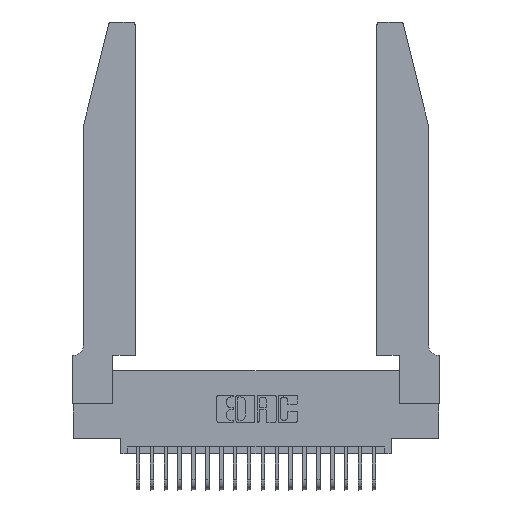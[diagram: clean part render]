
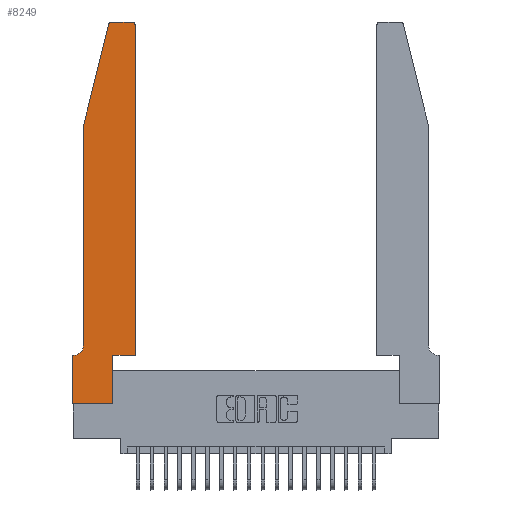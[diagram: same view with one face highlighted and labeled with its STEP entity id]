
A CAD part, top view. The second image highlights one B-rep face of the part: STEP entity #8249.
In plain terms, the highlighted planar face has unit normal (0, 0, 1).
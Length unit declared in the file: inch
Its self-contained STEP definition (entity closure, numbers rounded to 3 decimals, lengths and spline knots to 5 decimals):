
#25 = VERTEX_POINT ( 'NONE', #424 ) ;
#424 = CARTESIAN_POINT ( 'NONE',  ( 0.0055, 0.35, 0.37 ) ) ;
#788 = VERTEX_POINT ( 'NONE', #925 ) ;
#873 = EDGE_CURVE ( 'NONE', #8035, #13898, #9835, .T. ) ;
#921 = CARTESIAN_POINT ( 'NONE',  ( 0.2865, 0.35, 0.37 ) ) ;
#925 = CARTESIAN_POINT ( 'NONE',  ( 0.0755, 2., 0.37 ) ) ;
#930 = LINE ( 'NONE', #13418, #6035 ) ;
#1187 = ORIENTED_EDGE ( 'NONE', *, *, #9232, .T. ) ;
#1329 = DIRECTION ( 'NONE',  ( 0., 0., 1. ) ) ;
#1431 = EDGE_CURVE ( 'NONE', #19298, #11202, #3705, .T. ) ;
#1571 = CIRCLE ( 'NONE', #3192, 0.07 ) ;
#1923 = ORIENTED_EDGE ( 'NONE', *, *, #21018, .T. ) ;
#2057 = CARTESIAN_POINT ( 'NONE',  ( 0.4205, 2.75, 0.37 ) ) ;
#2669 = DIRECTION ( 'NONE',  ( 0., 1., 0. ) ) ;
#2806 = CARTESIAN_POINT ( 'NONE',  ( 0., 0.35, 0.37 ) ) ;
#3167 = VECTOR ( 'NONE', #20704, 39.37008 ) ;
#3180 = VERTEX_POINT ( 'NONE', #6716 ) ;
#3192 = AXIS2_PLACEMENT_3D ( 'NONE', #5181, #16887, #6897 ) ;
#3321 = DIRECTION ( 'NONE',  ( -1., 0., 0. ) ) ;
#3704 = CARTESIAN_POINT ( 'NONE',  ( 0.0755, 0.42, 0.37 ) ) ;
#3705 = LINE ( 'NONE', #14028, #3167 ) ;
#3751 = ORIENTED_EDGE ( 'NONE', *, *, #15415, .T. ) ;
#3829 = CARTESIAN_POINT ( 'NONE',  ( 0.4505, 0.35, 0.37 ) ) ;
#4126 = ORIENTED_EDGE ( 'NONE', *, *, #1431, .T. ) ;
#4267 = LINE ( 'NONE', #21011, #12687 ) ;
#4289 = DIRECTION ( 'NONE',  ( 0., 1., 0. ) ) ;
#4450 = AXIS2_PLACEMENT_3D ( 'NONE', #18983, #11532, #5230 ) ;
#4465 = CARTESIAN_POINT ( 'NONE',  ( 0., 0., 0.37 ) ) ;
#4555 = DIRECTION ( 'NONE',  ( 1., 0., 0. ) ) ;
#4570 = DIRECTION ( 'NONE',  ( 0., -1., 0. ) ) ;
#5181 = CARTESIAN_POINT ( 'NONE',  ( 0.0055, 0.42, 0.37 ) ) ;
#5230 = DIRECTION ( 'NONE',  ( 1., 0., 0. ) ) ;
#5267 = CARTESIAN_POINT ( 'NONE',  ( 0.0755, 0.35, 0.37 ) ) ;
#5274 = CARTESIAN_POINT ( 'NONE',  ( 0.284, 2.75, 0.37 ) ) ;
#6035 = VECTOR ( 'NONE', #3321, 39.37008 ) ;
#6087 = VERTEX_POINT ( 'NONE', #16178 ) ;
#6157 = DIRECTION ( 'NONE',  ( 0., -1., 0. ) ) ;
#6173 = PLANE ( 'NONE',  #8786 ) ;
#6716 = CARTESIAN_POINT ( 'NONE',  ( 0.2865, 0.35, 0.37 ) ) ;
#6897 = DIRECTION ( 'NONE',  ( -1., 0., 0. ) ) ;
#6988 = DIRECTION ( 'NONE',  ( -1., 0., 0. ) ) ;
#7423 = LINE ( 'NONE', #5267, #15754 ) ;
#7654 = VECTOR ( 'NONE', #6157, 39.37008 ) ;
#8035 = VERTEX_POINT ( 'NONE', #20699 ) ;
#8249 = ADVANCED_FACE ( 'NONE', ( #14577 ), #6173, .T. ) ;
#8595 = ORIENTED_EDGE ( 'NONE', *, *, #15744, .T. ) ;
#8786 = AXIS2_PLACEMENT_3D ( 'NONE', #2806, #14583, #4555 ) ;
#8890 = ORIENTED_EDGE ( 'NONE', *, *, #12503, .T. ) ;
#8979 = EDGE_CURVE ( 'NONE', #18994, #13188, #19507, .T. ) ;
#9232 = EDGE_CURVE ( 'NONE', #3180, #6087, #14841, .T. ) ;
#9474 = EDGE_CURVE ( 'NONE', #788, #10810, #11680, .T. ) ;
#9787 = VECTOR ( 'NONE', #2669, 39.37008 ) ;
#9819 = ORIENTED_EDGE ( 'NONE', *, *, #873, .T. ) ;
#9835 = CIRCLE ( 'NONE', #4450, 0.03 ) ;
#9926 = CARTESIAN_POINT ( 'NONE',  ( 0.0755, 2., 0.37 ) ) ;
#10230 = CARTESIAN_POINT ( 'NONE',  ( 0., 0.35, 0.37 ) ) ;
#10776 = LINE ( 'NONE', #9926, #18576 ) ;
#10810 = VERTEX_POINT ( 'NONE', #3704 ) ;
#11202 = VERTEX_POINT ( 'NONE', #19853 ) ;
#11277 = AXIS2_PLACEMENT_3D ( 'NONE', #11471, #1329, #13193 ) ;
#11471 = CARTESIAN_POINT ( 'NONE',  ( 0.284, 2.72, 0.37 ) ) ;
#11532 = DIRECTION ( 'NONE',  ( 0., 0., 1. ) ) ;
#11680 = LINE ( 'NONE', #21210, #19488 ) ;
#12456 = ORIENTED_EDGE ( 'NONE', *, *, #9474, .T. ) ;
#12503 = EDGE_CURVE ( 'NONE', #13188, #788, #10776, .T. ) ;
#12623 = ORIENTED_EDGE ( 'NONE', *, *, #21142, .T. ) ;
#12687 = VECTOR ( 'NONE', #4289, 39.37008 ) ;
#13188 = VERTEX_POINT ( 'NONE', #15335 ) ;
#13193 = DIRECTION ( 'NONE',  ( 1., 0., 0. ) ) ;
#13418 = CARTESIAN_POINT ( 'NONE',  ( 0.2605, 2.75, 0.37 ) ) ;
#13898 = VERTEX_POINT ( 'NONE', #2057 ) ;
#13903 = DIRECTION ( 'NONE',  ( 1., 0., 0. ) ) ;
#14028 = CARTESIAN_POINT ( 'NONE',  ( 0., 0., 0.37 ) ) ;
#14328 = CARTESIAN_POINT ( 'NONE',  ( 0., 0., 0.37 ) ) ;
#14577 = FACE_OUTER_BOUND ( 'NONE', #16951, .T. ) ;
#14583 = DIRECTION ( 'NONE',  ( 0., 0., 1. ) ) ;
#14841 = LINE ( 'NONE', #3829, #19227 ) ;
#15335 = CARTESIAN_POINT ( 'NONE',  ( 0.25487, 2.72718, 0.37 ) ) ;
#15415 = EDGE_CURVE ( 'NONE', #10810, #25, #1571, .T. ) ;
#15744 = EDGE_CURVE ( 'NONE', #6087, #8035, #4267, .T. ) ;
#15754 = VECTOR ( 'NONE', #6988, 39.37008 ) ;
#16178 = CARTESIAN_POINT ( 'NONE',  ( 0.4505, 0.35, 0.37 ) ) ;
#16887 = DIRECTION ( 'NONE',  ( 0., 0., -1. ) ) ;
#16951 = EDGE_LOOP ( 'NONE', ( #12623, #20674, #8890, #12456, #3751, #19215, #1923, #4126, #17241, #1187, #8595, #9819 ) ) ;
#17241 = ORIENTED_EDGE ( 'NONE', *, *, #19992, .T. ) ;
#18576 = VECTOR ( 'NONE', #19873, 39.37008 ) ;
#18599 = LINE ( 'NONE', #921, #9787 ) ;
#18983 = CARTESIAN_POINT ( 'NONE',  ( 0.4205, 2.72, 0.37 ) ) ;
#18994 = VERTEX_POINT ( 'NONE', #5274 ) ;
#19215 = ORIENTED_EDGE ( 'NONE', *, *, #20376, .T. ) ;
#19227 = VECTOR ( 'NONE', #13903, 39.37008 ) ;
#19298 = VERTEX_POINT ( 'NONE', #14328 ) ;
#19488 = VECTOR ( 'NONE', #4570, 39.37008 ) ;
#19507 = CIRCLE ( 'NONE', #11277, 0.03 ) ;
#19624 = VERTEX_POINT ( 'NONE', #10230 ) ;
#19853 = CARTESIAN_POINT ( 'NONE',  ( 0.2865, 0., 0.37 ) ) ;
#19873 = DIRECTION ( 'NONE',  ( -0.239, -0.971, 0. ) ) ;
#19992 = EDGE_CURVE ( 'NONE', #11202, #3180, #18599, .T. ) ;
#20376 = EDGE_CURVE ( 'NONE', #25, #19624, #7423, .T. ) ;
#20674 = ORIENTED_EDGE ( 'NONE', *, *, #8979, .T. ) ;
#20699 = CARTESIAN_POINT ( 'NONE',  ( 0.4505, 2.72, 0.37 ) ) ;
#20704 = DIRECTION ( 'NONE',  ( 1., 0., 0. ) ) ;
#20911 = LINE ( 'NONE', #4465, #7654 ) ;
#21011 = CARTESIAN_POINT ( 'NONE',  ( 0.4505, 0.35, 0.37 ) ) ;
#21018 = EDGE_CURVE ( 'NONE', #19624, #19298, #20911, .T. ) ;
#21142 = EDGE_CURVE ( 'NONE', #13898, #18994, #930, .T. ) ;
#21210 = CARTESIAN_POINT ( 'NONE',  ( 0.0755, 2., 0.37 ) ) ;
